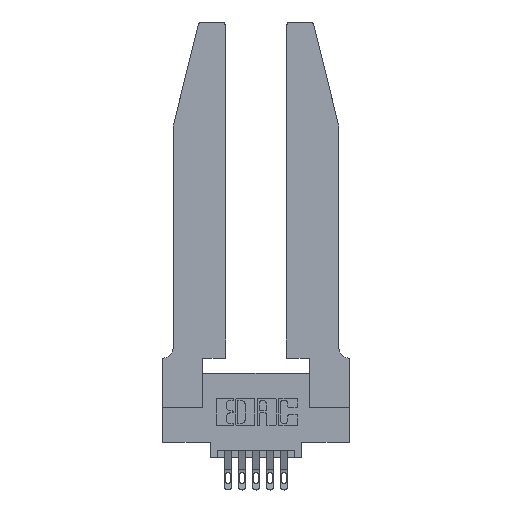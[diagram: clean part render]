
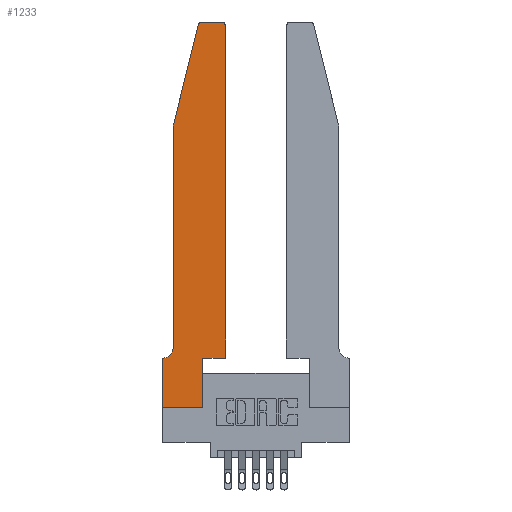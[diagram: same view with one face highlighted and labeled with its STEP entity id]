
A CAD part, top view. The second image highlights one B-rep face of the part: STEP entity #1233.
In plain terms, the highlighted planar face has unit normal (0, 0, 1).
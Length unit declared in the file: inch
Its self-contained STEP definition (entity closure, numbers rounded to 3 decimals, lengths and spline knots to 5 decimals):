
#33 = CARTESIAN_POINT ( 'NONE',  ( 0.4505, 0.35, 0.37 ) ) ;
#73 = ORIENTED_EDGE ( 'NONE', *, *, #13687, .T. ) ;
#169 = VERTEX_POINT ( 'NONE', #1166 ) ;
#179 = LINE ( 'NONE', #12937, #2883 ) ;
#454 = VECTOR ( 'NONE', #3810, 39.37008 ) ;
#491 = VECTOR ( 'NONE', #9685, 39.37008 ) ;
#574 = DIRECTION ( 'NONE',  ( 0., 1., 0. ) ) ;
#701 = CARTESIAN_POINT ( 'NONE',  ( 0.2605, 2.75, 0.37 ) ) ;
#758 = CARTESIAN_POINT ( 'NONE',  ( 0.0055, 0.42, 0.37 ) ) ;
#844 = VECTOR ( 'NONE', #6371, 39.37008 ) ;
#913 = CARTESIAN_POINT ( 'NONE',  ( 0., 0., 0.37 ) ) ;
#923 = ORIENTED_EDGE ( 'NONE', *, *, #13136, .T. ) ;
#1166 = CARTESIAN_POINT ( 'NONE',  ( 0.0055, 0.35, 0.37 ) ) ;
#1232 = LINE ( 'NONE', #10610, #844 ) ;
#1233 = ADVANCED_FACE ( 'NONE', ( #11385 ), #5696, .T. ) ;
#1268 = LINE ( 'NONE', #9449, #12148 ) ;
#1331 = CARTESIAN_POINT ( 'NONE',  ( 0.4505, 0.35, 0.37 ) ) ;
#1446 = CARTESIAN_POINT ( 'NONE',  ( 0.2865, 0., 0.37 ) ) ;
#1513 = EDGE_LOOP ( 'NONE', ( #12298, #10870, #3216, #5574, #9578, #923, #73, #7165, #2389, #3687, #6540, #3414 ) ) ;
#1735 = CARTESIAN_POINT ( 'NONE',  ( 0., 0., 0.37 ) ) ;
#1870 = VERTEX_POINT ( 'NONE', #9749 ) ;
#1911 = DIRECTION ( 'NONE',  ( -1., 0., 0. ) ) ;
#1946 = CIRCLE ( 'NONE', #5640, 0.03 ) ;
#1993 = CARTESIAN_POINT ( 'NONE',  ( 0.284, 2.75, 0.37 ) ) ;
#2086 = CARTESIAN_POINT ( 'NONE',  ( 0.4205, 2.72, 0.37 ) ) ;
#2382 = DIRECTION ( 'NONE',  ( 1., 0., 0. ) ) ;
#2389 = ORIENTED_EDGE ( 'NONE', *, *, #9279, .T. ) ;
#2883 = VECTOR ( 'NONE', #4406, 39.37008 ) ;
#3213 = DIRECTION ( 'NONE',  ( 1., 0., 0. ) ) ;
#3216 = ORIENTED_EDGE ( 'NONE', *, *, #11138, .T. ) ;
#3414 = ORIENTED_EDGE ( 'NONE', *, *, #8814, .T. ) ;
#3494 = LINE ( 'NONE', #11308, #454 ) ;
#3618 = VERTEX_POINT ( 'NONE', #1446 ) ;
#3687 = ORIENTED_EDGE ( 'NONE', *, *, #3958, .T. ) ;
#3789 = VERTEX_POINT ( 'NONE', #1735 ) ;
#3810 = DIRECTION ( 'NONE',  ( -0.239, -0.971, 0. ) ) ;
#3958 = EDGE_CURVE ( 'NONE', #12129, #13524, #4636, .T. ) ;
#4024 = VERTEX_POINT ( 'NONE', #4748 ) ;
#4059 = CARTESIAN_POINT ( 'NONE',  ( 0.2865, 0.35, 0.37 ) ) ;
#4152 = DIRECTION ( 'NONE',  ( 0., 0., 1. ) ) ;
#4406 = DIRECTION ( 'NONE',  ( 0., 1., 0. ) ) ;
#4636 = LINE ( 'NONE', #33, #12800 ) ;
#4748 = CARTESIAN_POINT ( 'NONE',  ( 0.4205, 2.75, 0.37 ) ) ;
#4758 = CARTESIAN_POINT ( 'NONE',  ( 0., 0.35, 0.37 ) ) ;
#4776 = VERTEX_POINT ( 'NONE', #13440 ) ;
#4921 = CIRCLE ( 'NONE', #12846, 0.07 ) ;
#5291 = LINE ( 'NONE', #701, #5637 ) ;
#5574 = ORIENTED_EDGE ( 'NONE', *, *, #9390, .T. ) ;
#5637 = VECTOR ( 'NONE', #9489, 39.37008 ) ;
#5640 = AXIS2_PLACEMENT_3D ( 'NONE', #2086, #9699, #3213 ) ;
#5696 = PLANE ( 'NONE',  #11650 ) ;
#5716 = DIRECTION ( 'NONE',  ( 0., 0., 1. ) ) ;
#5904 = EDGE_CURVE ( 'NONE', #1870, #169, #4921, .T. ) ;
#6068 = CARTESIAN_POINT ( 'NONE',  ( 0., 0.35, 0.37 ) ) ;
#6371 = DIRECTION ( 'NONE',  ( 0., -1., 0. ) ) ;
#6498 = DIRECTION ( 'NONE',  ( 0., -1., 0. ) ) ;
#6540 = ORIENTED_EDGE ( 'NONE', *, *, #7016, .T. ) ;
#6853 = CIRCLE ( 'NONE', #11962, 0.03 ) ;
#7016 = EDGE_CURVE ( 'NONE', #13524, #12859, #179, .T. ) ;
#7165 = ORIENTED_EDGE ( 'NONE', *, *, #9466, .T. ) ;
#7414 = EDGE_CURVE ( 'NONE', #12504, #4776, #6853, .T. ) ;
#7502 = VECTOR ( 'NONE', #8624, 39.37008 ) ;
#7553 = CARTESIAN_POINT ( 'NONE',  ( 0.0755, 0.35, 0.37 ) ) ;
#8272 = EDGE_CURVE ( 'NONE', #4024, #12504, #5291, .T. ) ;
#8456 = LINE ( 'NONE', #4059, #13430 ) ;
#8485 = DIRECTION ( 'NONE',  ( 0., 0., -1. ) ) ;
#8624 = DIRECTION ( 'NONE',  ( -1., 0., 0. ) ) ;
#8814 = EDGE_CURVE ( 'NONE', #12859, #4024, #1946, .T. ) ;
#8900 = VERTEX_POINT ( 'NONE', #11941 ) ;
#9279 = EDGE_CURVE ( 'NONE', #3618, #12129, #8456, .T. ) ;
#9363 = DIRECTION ( 'NONE',  ( 1., 0., 0. ) ) ;
#9390 = EDGE_CURVE ( 'NONE', #8900, #1870, #1232, .T. ) ;
#9449 = CARTESIAN_POINT ( 'NONE',  ( 0., 0., 0.37 ) ) ;
#9466 = EDGE_CURVE ( 'NONE', #3789, #3618, #11436, .T. ) ;
#9489 = DIRECTION ( 'NONE',  ( -1., 0., 0. ) ) ;
#9578 = ORIENTED_EDGE ( 'NONE', *, *, #5904, .T. ) ;
#9685 = DIRECTION ( 'NONE',  ( 1., 0., 0. ) ) ;
#9699 = DIRECTION ( 'NONE',  ( 0., 0., 1. ) ) ;
#9749 = CARTESIAN_POINT ( 'NONE',  ( 0.0755, 0.42, 0.37 ) ) ;
#10302 = VERTEX_POINT ( 'NONE', #4758 ) ;
#10551 = CARTESIAN_POINT ( 'NONE',  ( 0.284, 2.72, 0.37 ) ) ;
#10610 = CARTESIAN_POINT ( 'NONE',  ( 0.0755, 2., 0.37 ) ) ;
#10870 = ORIENTED_EDGE ( 'NONE', *, *, #7414, .T. ) ;
#11138 = EDGE_CURVE ( 'NONE', #4776, #8900, #3494, .T. ) ;
#11308 = CARTESIAN_POINT ( 'NONE',  ( 0.0755, 2., 0.37 ) ) ;
#11385 = FACE_OUTER_BOUND ( 'NONE', #1513, .T. ) ;
#11436 = LINE ( 'NONE', #913, #491 ) ;
#11639 = DIRECTION ( 'NONE',  ( 1., 0., 0. ) ) ;
#11650 = AXIS2_PLACEMENT_3D ( 'NONE', #6068, #5716, #9363 ) ;
#11941 = CARTESIAN_POINT ( 'NONE',  ( 0.0755, 2., 0.37 ) ) ;
#11962 = AXIS2_PLACEMENT_3D ( 'NONE', #10551, #4152, #11639 ) ;
#12129 = VERTEX_POINT ( 'NONE', #13195 ) ;
#12148 = VECTOR ( 'NONE', #6498, 39.37008 ) ;
#12298 = ORIENTED_EDGE ( 'NONE', *, *, #8272, .T. ) ;
#12504 = VERTEX_POINT ( 'NONE', #1993 ) ;
#12800 = VECTOR ( 'NONE', #2382, 39.37008 ) ;
#12846 = AXIS2_PLACEMENT_3D ( 'NONE', #758, #8485, #1911 ) ;
#12859 = VERTEX_POINT ( 'NONE', #13460 ) ;
#12937 = CARTESIAN_POINT ( 'NONE',  ( 0.4505, 0.35, 0.37 ) ) ;
#13136 = EDGE_CURVE ( 'NONE', #169, #10302, #13138, .T. ) ;
#13138 = LINE ( 'NONE', #7553, #7502 ) ;
#13195 = CARTESIAN_POINT ( 'NONE',  ( 0.2865, 0.35, 0.37 ) ) ;
#13430 = VECTOR ( 'NONE', #574, 39.37008 ) ;
#13440 = CARTESIAN_POINT ( 'NONE',  ( 0.25487, 2.72718, 0.37 ) ) ;
#13460 = CARTESIAN_POINT ( 'NONE',  ( 0.4505, 2.72, 0.37 ) ) ;
#13524 = VERTEX_POINT ( 'NONE', #1331 ) ;
#13687 = EDGE_CURVE ( 'NONE', #10302, #3789, #1268, .T. ) ;
